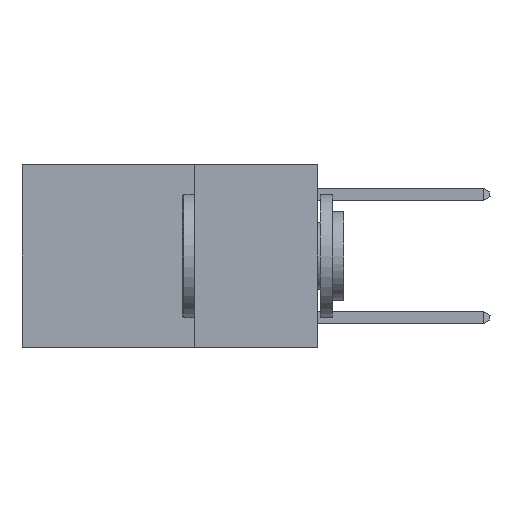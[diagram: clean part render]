
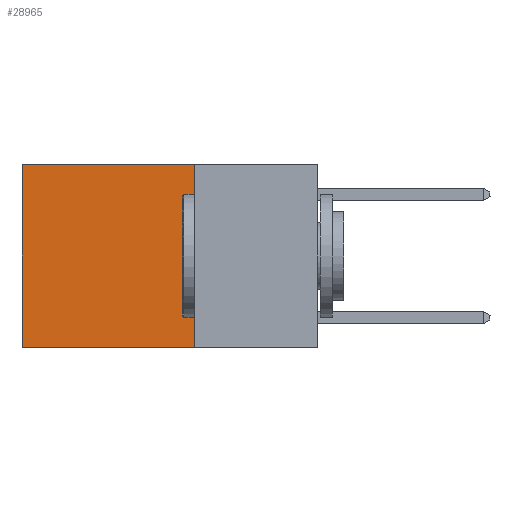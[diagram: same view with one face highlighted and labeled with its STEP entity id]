
A CAD part, left-side view. The second image highlights one B-rep face of the part: STEP entity #28965.
In plain terms, the highlighted planar face has unit normal (-1, 0, 0).
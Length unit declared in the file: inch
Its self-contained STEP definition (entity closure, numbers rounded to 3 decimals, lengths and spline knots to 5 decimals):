
#963 = VECTOR ( 'NONE', #31941, 39.37008 ) ;
#1595 = CARTESIAN_POINT ( 'NONE',  ( 0.2625, 0.25, 0. ) ) ;
#4042 = LINE ( 'NONE', #1595, #8999 ) ;
#4621 = CARTESIAN_POINT ( 'NONE',  ( 0.2625, 0.25, 0. ) ) ;
#5393 = DIRECTION ( 'NONE',  ( 0., 1., 0. ) ) ;
#6496 = EDGE_LOOP ( 'NONE', ( #25123, #16565, #22045, #22948 ) ) ;
#6931 = CARTESIAN_POINT ( 'NONE',  ( 0.2625, 0.6, -0.37 ) ) ;
#8195 = DIRECTION ( 'NONE',  ( 0., 0., -1. ) ) ;
#8275 = VECTOR ( 'NONE', #18321, 39.37008 ) ;
#8528 = VERTEX_POINT ( 'NONE', #19042 ) ;
#8999 = VECTOR ( 'NONE', #9100, 39.37008 ) ;
#9100 = DIRECTION ( 'NONE',  ( 0., 0., -1. ) ) ;
#10641 = CARTESIAN_POINT ( 'NONE',  ( 0.2625, 0.25, 0. ) ) ;
#10963 = DIRECTION ( 'NONE',  ( 1., 0., 0. ) ) ;
#11003 = VERTEX_POINT ( 'NONE', #25234 ) ;
#12443 = AXIS2_PLACEMENT_3D ( 'NONE', #10641, #10963, #8195 ) ;
#13099 = LINE ( 'NONE', #23022, #8275 ) ;
#13574 = FACE_OUTER_BOUND ( 'NONE', #6496, .T. ) ;
#15059 = VERTEX_POINT ( 'NONE', #4621 ) ;
#16565 = ORIENTED_EDGE ( 'NONE', *, *, #28952, .F. ) ;
#17413 = EDGE_CURVE ( 'NONE', #15059, #11003, #4042, .T. ) ;
#18009 = PLANE ( 'NONE',  #12443 ) ;
#18321 = DIRECTION ( 'NONE',  ( 0., 1., 0. ) ) ;
#19042 = CARTESIAN_POINT ( 'NONE',  ( 0.2625, 0.6, 0. ) ) ;
#19913 = CARTESIAN_POINT ( 'NONE',  ( 0.2625, 0.6, 0. ) ) ;
#21856 = LINE ( 'NONE', #19913, #963 ) ;
#22045 = ORIENTED_EDGE ( 'NONE', *, *, #17413, .F. ) ;
#22948 = ORIENTED_EDGE ( 'NONE', *, *, #29454, .T. ) ;
#23022 = CARTESIAN_POINT ( 'NONE',  ( 0.2625, 0.25, -0.37 ) ) ;
#23278 = CARTESIAN_POINT ( 'NONE',  ( 0.2625, 0.25, 0. ) ) ;
#23887 = VECTOR ( 'NONE', #5393, 39.37008 ) ;
#25123 = ORIENTED_EDGE ( 'NONE', *, *, #28238, .T. ) ;
#25234 = CARTESIAN_POINT ( 'NONE',  ( 0.2625, 0.25, -0.37 ) ) ;
#27837 = LINE ( 'NONE', #23278, #23887 ) ;
#28238 = EDGE_CURVE ( 'NONE', #8528, #29994, #21856, .T. ) ;
#28952 = EDGE_CURVE ( 'NONE', #11003, #29994, #13099, .T. ) ;
#28965 = ADVANCED_FACE ( 'NONE', ( #13574 ), #18009, .F. ) ;
#29454 = EDGE_CURVE ( 'NONE', #15059, #8528, #27837, .T. ) ;
#29994 = VERTEX_POINT ( 'NONE', #6931 ) ;
#31941 = DIRECTION ( 'NONE',  ( 0., 0., -1. ) ) ;
